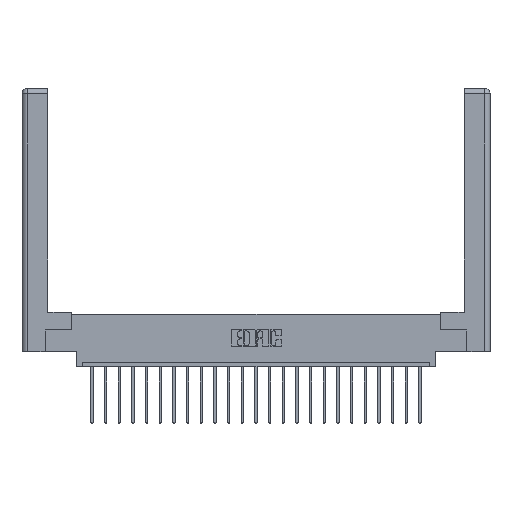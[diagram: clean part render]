
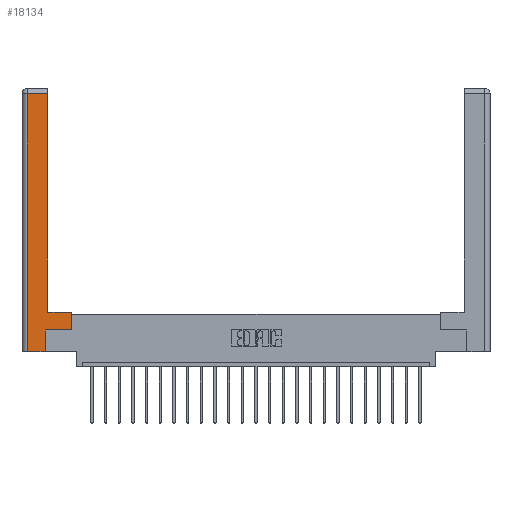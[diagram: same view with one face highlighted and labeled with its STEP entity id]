
A CAD part, top view. The second image highlights one B-rep face of the part: STEP entity #18134.
In plain terms, the highlighted planar face has unit normal (0, 0, 1).
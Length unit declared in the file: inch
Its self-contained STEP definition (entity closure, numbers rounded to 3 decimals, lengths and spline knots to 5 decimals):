
#565 = LINE ( 'NONE', #2199, #19365 ) ;
#756 = VERTEX_POINT ( 'NONE', #18886 ) ;
#983 = ORIENTED_EDGE ( 'NONE', *, *, #7029, .T. ) ;
#1012 = DIRECTION ( 'NONE',  ( 0., 1., 0. ) ) ;
#1175 = VERTEX_POINT ( 'NONE', #9658 ) ;
#2029 = CARTESIAN_POINT ( 'NONE',  ( 0.295, 0.45, 0. ) ) ;
#2083 = EDGE_CURVE ( 'NONE', #15446, #17124, #19896, .T. ) ;
#2199 = CARTESIAN_POINT ( 'NONE',  ( 0.565, 0.245, 0. ) ) ;
#2517 = VECTOR ( 'NONE', #21578, 39.37008 ) ;
#2932 = ORIENTED_EDGE ( 'NONE', *, *, #21739, .T. ) ;
#3039 = EDGE_CURVE ( 'NONE', #756, #15446, #9891, .T. ) ;
#3396 = VECTOR ( 'NONE', #1012, 39.37008 ) ;
#3717 = VERTEX_POINT ( 'NONE', #23235 ) ;
#4306 = VERTEX_POINT ( 'NONE', #16080 ) ;
#4399 = VECTOR ( 'NONE', #6302, 39.37008 ) ;
#5306 = CARTESIAN_POINT ( 'NONE',  ( 0.565, 0.45, 0. ) ) ;
#6302 = DIRECTION ( 'NONE',  ( 0., 1., 0. ) ) ;
#6699 = VERTEX_POINT ( 'NONE', #10432 ) ;
#7029 = EDGE_CURVE ( 'NONE', #4306, #21177, #7907, .T. ) ;
#7907 = LINE ( 'NONE', #15403, #3396 ) ;
#7911 = VECTOR ( 'NONE', #21516, 39.37008 ) ;
#7922 = AXIS2_PLACEMENT_3D ( 'NONE', #10234, #8334, #23425 ) ;
#8334 = DIRECTION ( 'NONE',  ( 0., 0., -1. ) ) ;
#8390 = ORIENTED_EDGE ( 'NONE', *, *, #19779, .T. ) ;
#8520 = CARTESIAN_POINT ( 'NONE',  ( 0.295, 0.45, 0. ) ) ;
#8561 = LINE ( 'NONE', #19993, #21070 ) ;
#8885 = CARTESIAN_POINT ( 'NONE',  ( 0.0615, 2.94, 0. ) ) ;
#9058 = DIRECTION ( 'NONE',  ( -1., 0., 0. ) ) ;
#9658 = CARTESIAN_POINT ( 'NONE',  ( 0.0615, 2.94, 0. ) ) ;
#9891 = LINE ( 'NONE', #5306, #7911 ) ;
#10045 = ORIENTED_EDGE ( 'NONE', *, *, #3039, .T. ) ;
#10234 = CARTESIAN_POINT ( 'NONE',  ( 0., 0., 0. ) ) ;
#10307 = ORIENTED_EDGE ( 'NONE', *, *, #21843, .T. ) ;
#10432 = CARTESIAN_POINT ( 'NONE',  ( 0.0615, 0., 0. ) ) ;
#11204 = LINE ( 'NONE', #12541, #4399 ) ;
#11444 = FACE_OUTER_BOUND ( 'NONE', #20607, .T. ) ;
#12541 = CARTESIAN_POINT ( 'NONE',  ( 0.295, 3., 0. ) ) ;
#12809 = DIRECTION ( 'NONE',  ( 1., 0., 0. ) ) ;
#12901 = EDGE_CURVE ( 'NONE', #17124, #3717, #11204, .T. ) ;
#13447 = LINE ( 'NONE', #13908, #15453 ) ;
#13455 = ORIENTED_EDGE ( 'NONE', *, *, #12901, .T. ) ;
#13908 = CARTESIAN_POINT ( 'NONE',  ( 0.0615, 0., 0. ) ) ;
#15403 = CARTESIAN_POINT ( 'NONE',  ( 0.265, 0.245, 0. ) ) ;
#15446 = VERTEX_POINT ( 'NONE', #19540 ) ;
#15453 = VECTOR ( 'NONE', #15778, 39.37008 ) ;
#15778 = DIRECTION ( 'NONE',  ( 0., -1., 0. ) ) ;
#16016 = PLANE ( 'NONE',  #7922 ) ;
#16080 = CARTESIAN_POINT ( 'NONE',  ( 0.265, 0., 0. ) ) ;
#16523 = ORIENTED_EDGE ( 'NONE', *, *, #22790, .T. ) ;
#17124 = VERTEX_POINT ( 'NONE', #8520 ) ;
#18057 = ORIENTED_EDGE ( 'NONE', *, *, #2083, .T. ) ;
#18134 = ADVANCED_FACE ( 'NONE', ( #11444 ), #16016, .F. ) ;
#18886 = CARTESIAN_POINT ( 'NONE',  ( 0.565, 0.245, 0. ) ) ;
#19365 = VECTOR ( 'NONE', #22241, 39.37008 ) ;
#19540 = CARTESIAN_POINT ( 'NONE',  ( 0.565, 0.45, 0. ) ) ;
#19779 = EDGE_CURVE ( 'NONE', #1175, #6699, #13447, .T. ) ;
#19896 = LINE ( 'NONE', #2029, #20442 ) ;
#19993 = CARTESIAN_POINT ( 'NONE',  ( 0.265, 0., 0. ) ) ;
#20442 = VECTOR ( 'NONE', #9058, 39.37008 ) ;
#20607 = EDGE_LOOP ( 'NONE', ( #13455, #16523, #8390, #2932, #983, #10307, #10045, #18057 ) ) ;
#20750 = LINE ( 'NONE', #8885, #2517 ) ;
#21070 = VECTOR ( 'NONE', #12809, 39.37008 ) ;
#21177 = VERTEX_POINT ( 'NONE', #22272 ) ;
#21516 = DIRECTION ( 'NONE',  ( 0., 1., 0. ) ) ;
#21578 = DIRECTION ( 'NONE',  ( -1., 0., 0. ) ) ;
#21739 = EDGE_CURVE ( 'NONE', #6699, #4306, #8561, .T. ) ;
#21843 = EDGE_CURVE ( 'NONE', #21177, #756, #565, .T. ) ;
#22241 = DIRECTION ( 'NONE',  ( 1., 0., 0. ) ) ;
#22272 = CARTESIAN_POINT ( 'NONE',  ( 0.265, 0.245, 0. ) ) ;
#22790 = EDGE_CURVE ( 'NONE', #3717, #1175, #20750, .T. ) ;
#23235 = CARTESIAN_POINT ( 'NONE',  ( 0.295, 2.94, 0. ) ) ;
#23425 = DIRECTION ( 'NONE',  ( -1., 0., 0. ) ) ;
